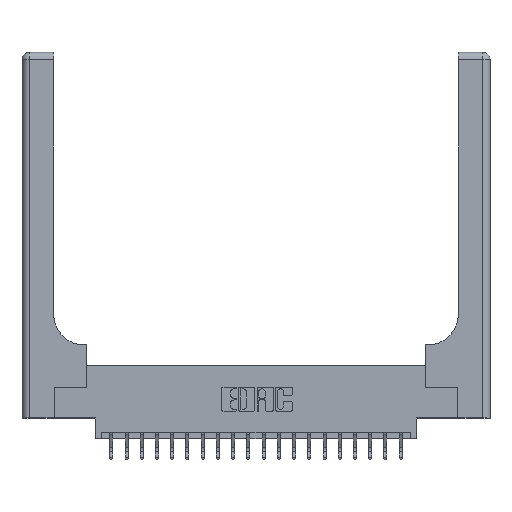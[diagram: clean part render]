
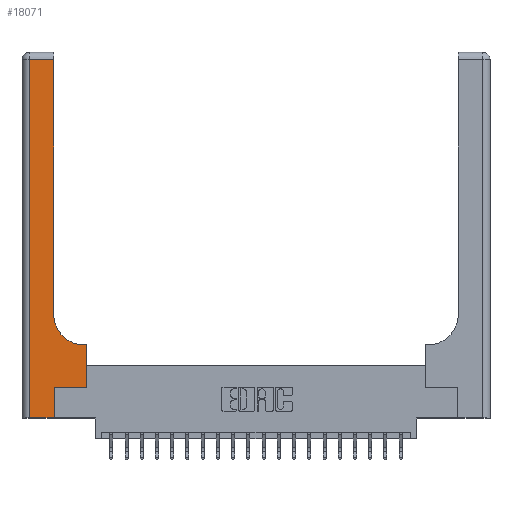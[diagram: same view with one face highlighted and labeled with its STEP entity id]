
A CAD part, top view. The second image highlights one B-rep face of the part: STEP entity #18071.
In plain terms, the highlighted planar face has unit normal (0, 0, 1).
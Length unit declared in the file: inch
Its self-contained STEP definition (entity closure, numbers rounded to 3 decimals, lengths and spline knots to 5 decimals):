
#73 = LINE ( 'NONE', #6132, #603 ) ;
#292 = EDGE_CURVE ( 'NONE', #10400, #18413, #14220, .T. ) ;
#494 = LINE ( 'NONE', #15531, #1021 ) ;
#603 = VECTOR ( 'NONE', #17720, 39.37008 ) ;
#680 = ORIENTED_EDGE ( 'NONE', *, *, #18925, .T. ) ;
#1021 = VECTOR ( 'NONE', #5498, 39.37008 ) ;
#1068 = CARTESIAN_POINT ( 'NONE',  ( 0.265, 0.25, 0.37 ) ) ;
#1301 = CIRCLE ( 'NONE', #16446, 0.25 ) ;
#1628 = EDGE_LOOP ( 'NONE', ( #680, #21188, #3994, #5048, #20464, #15556, #20188, #12315, #20266 ) ) ;
#1941 = CARTESIAN_POINT ( 'NONE',  ( 0.265, 0., 0.37 ) ) ;
#2026 = EDGE_CURVE ( 'NONE', #15609, #5024, #1301, .T. ) ;
#2072 = CARTESIAN_POINT ( 'NONE',  ( 0.51, 0.85, 0.37 ) ) ;
#3595 = LINE ( 'NONE', #9870, #11991 ) ;
#3776 = DIRECTION ( 'NONE',  ( 1., 0., 0. ) ) ;
#3994 = ORIENTED_EDGE ( 'NONE', *, *, #19865, .T. ) ;
#4571 = FACE_OUTER_BOUND ( 'NONE', #1628, .T. ) ;
#5024 = VERTEX_POINT ( 'NONE', #18238 ) ;
#5048 = ORIENTED_EDGE ( 'NONE', *, *, #9239, .T. ) ;
#5498 = DIRECTION ( 'NONE',  ( 1., 0., 0. ) ) ;
#6132 = CARTESIAN_POINT ( 'NONE',  ( 0.26, 0.6, 0.37 ) ) ;
#6455 = VERTEX_POINT ( 'NONE', #6840 ) ;
#6603 = CARTESIAN_POINT ( 'NONE',  ( 0., 2.94, 0.37 ) ) ;
#6840 = CARTESIAN_POINT ( 'NONE',  ( 0.26, 2.94, 0.37 ) ) ;
#7053 = VERTEX_POINT ( 'NONE', #14000 ) ;
#7057 = VECTOR ( 'NONE', #18301, 39.37008 ) ;
#7759 = CARTESIAN_POINT ( 'NONE',  ( 0.265, 0., 0.37 ) ) ;
#8197 = VERTEX_POINT ( 'NONE', #14890 ) ;
#8418 = CARTESIAN_POINT ( 'NONE',  ( 0., 3., 0.37 ) ) ;
#8497 = DIRECTION ( 'NONE',  ( 0., 0., -1. ) ) ;
#9239 = EDGE_CURVE ( 'NONE', #16023, #10400, #494, .T. ) ;
#9244 = VECTOR ( 'NONE', #16118, 39.37008 ) ;
#9832 = CARTESIAN_POINT ( 'NONE',  ( 0.06, 3., 0.37 ) ) ;
#9870 = CARTESIAN_POINT ( 'NONE',  ( 0.528, 0.25, 0.37 ) ) ;
#9989 = VECTOR ( 'NONE', #16440, 39.37008 ) ;
#10400 = VERTEX_POINT ( 'NONE', #1941 ) ;
#10826 = CARTESIAN_POINT ( 'NONE',  ( 0.26, 3., 0.37 ) ) ;
#10981 = CARTESIAN_POINT ( 'NONE',  ( 0.06, 2.94, 0.37 ) ) ;
#11551 = DIRECTION ( 'NONE',  ( 0., 1., 0. ) ) ;
#11829 = VECTOR ( 'NONE', #18943, 39.37008 ) ;
#11991 = VECTOR ( 'NONE', #11551, 39.37008 ) ;
#12315 = ORIENTED_EDGE ( 'NONE', *, *, #20535, .T. ) ;
#12374 = AXIS2_PLACEMENT_3D ( 'NONE', #8418, #8497, #20059 ) ;
#13816 = DIRECTION ( 'NONE',  ( 0., 0., -1. ) ) ;
#13956 = CARTESIAN_POINT ( 'NONE',  ( 0.06, 0., 0.37 ) ) ;
#14000 = CARTESIAN_POINT ( 'NONE',  ( 0.528, 0.25, 0.37 ) ) ;
#14220 = LINE ( 'NONE', #7759, #9244 ) ;
#14401 = EDGE_CURVE ( 'NONE', #6455, #20473, #20815, .T. ) ;
#14890 = CARTESIAN_POINT ( 'NONE',  ( 0.528, 0.6, 0.37 ) ) ;
#14986 = VECTOR ( 'NONE', #20698, 39.37008 ) ;
#15531 = CARTESIAN_POINT ( 'NONE',  ( 0., 0., 0.37 ) ) ;
#15556 = ORIENTED_EDGE ( 'NONE', *, *, #19546, .T. ) ;
#15609 = VERTEX_POINT ( 'NONE', #16131 ) ;
#15728 = EDGE_CURVE ( 'NONE', #7053, #8197, #3595, .T. ) ;
#16023 = VERTEX_POINT ( 'NONE', #13956 ) ;
#16118 = DIRECTION ( 'NONE',  ( 0., 1., 0. ) ) ;
#16131 = CARTESIAN_POINT ( 'NONE',  ( 0.51, 0.6, 0.37 ) ) ;
#16440 = DIRECTION ( 'NONE',  ( 0., -1., 0. ) ) ;
#16446 = AXIS2_PLACEMENT_3D ( 'NONE', #2072, #13816, #3776 ) ;
#16752 = LINE ( 'NONE', #17315, #11829 ) ;
#16803 = PLANE ( 'NONE',  #12374 ) ;
#17315 = CARTESIAN_POINT ( 'NONE',  ( 0.265, 0.25, 0.37 ) ) ;
#17720 = DIRECTION ( 'NONE',  ( -1., 0., 0. ) ) ;
#18071 = ADVANCED_FACE ( 'NONE', ( #4571 ), #16803, .F. ) ;
#18238 = CARTESIAN_POINT ( 'NONE',  ( 0.26, 0.85, 0.37 ) ) ;
#18301 = DIRECTION ( 'NONE',  ( -1., 0., 0. ) ) ;
#18413 = VERTEX_POINT ( 'NONE', #1068 ) ;
#18763 = LINE ( 'NONE', #9832, #9989 ) ;
#18925 = EDGE_CURVE ( 'NONE', #5024, #6455, #19330, .T. ) ;
#18943 = DIRECTION ( 'NONE',  ( 1., 0., 0. ) ) ;
#19330 = LINE ( 'NONE', #10826, #14986 ) ;
#19546 = EDGE_CURVE ( 'NONE', #18413, #7053, #16752, .T. ) ;
#19865 = EDGE_CURVE ( 'NONE', #20473, #16023, #18763, .T. ) ;
#20059 = DIRECTION ( 'NONE',  ( -1., 0., 0. ) ) ;
#20188 = ORIENTED_EDGE ( 'NONE', *, *, #15728, .T. ) ;
#20266 = ORIENTED_EDGE ( 'NONE', *, *, #2026, .T. ) ;
#20464 = ORIENTED_EDGE ( 'NONE', *, *, #292, .T. ) ;
#20473 = VERTEX_POINT ( 'NONE', #10981 ) ;
#20535 = EDGE_CURVE ( 'NONE', #8197, #15609, #73, .T. ) ;
#20698 = DIRECTION ( 'NONE',  ( 0., 1., 0. ) ) ;
#20815 = LINE ( 'NONE', #6603, #7057 ) ;
#21188 = ORIENTED_EDGE ( 'NONE', *, *, #14401, .T. ) ;
